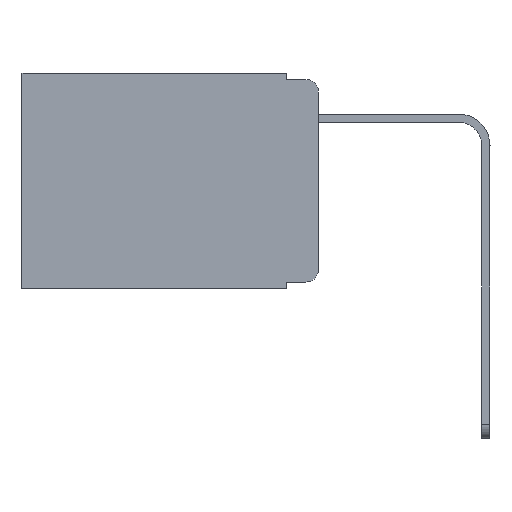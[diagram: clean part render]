
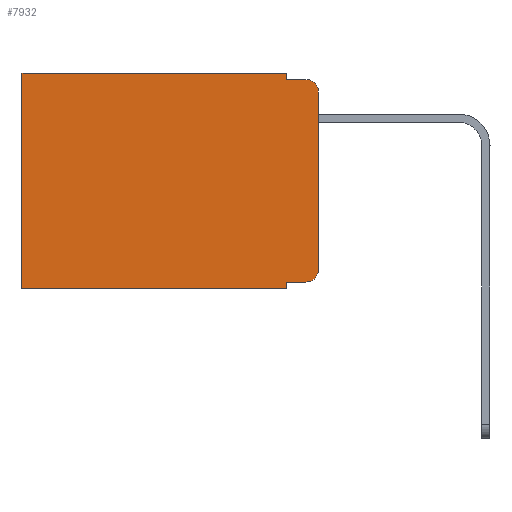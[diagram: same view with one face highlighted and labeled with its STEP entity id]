
A CAD part, left-side view. The second image highlights one B-rep face of the part: STEP entity #7932.
In plain terms, the highlighted planar face has unit normal (-1, 0, 0).
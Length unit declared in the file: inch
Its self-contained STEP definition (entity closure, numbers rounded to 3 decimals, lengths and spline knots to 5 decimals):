
#112 = EDGE_LOOP ( 'NONE', ( #2120, #5656, #2604, #1075, #7360, #4622, #6411, #9965, #1761, #8340 ) ) ;
#137 = DIRECTION ( 'NONE',  ( -1., 0., 0. ) ) ;
#188 = CARTESIAN_POINT ( 'NONE',  ( 0.298, 0.051, -0.333 ) ) ;
#479 = VERTEX_POINT ( 'NONE', #3732 ) ;
#549 = CARTESIAN_POINT ( 'NONE',  ( 0.298, 0.051, -0.01 ) ) ;
#800 = VERTEX_POINT ( 'NONE', #10415 ) ;
#1061 = LINE ( 'NONE', #8242, #6651 ) ;
#1075 = ORIENTED_EDGE ( 'NONE', *, *, #8992, .F. ) ;
#1256 = EDGE_CURVE ( 'NONE', #8599, #2444, #7581, .T. ) ;
#1360 = VERTEX_POINT ( 'NONE', #4017 ) ;
#1378 = AXIS2_PLACEMENT_3D ( 'NONE', #6893, #1524, #9546 ) ;
#1464 = LINE ( 'NONE', #3446, #11587 ) ;
#1524 = DIRECTION ( 'NONE',  ( -1., 0., 0. ) ) ;
#1761 = ORIENTED_EDGE ( 'NONE', *, *, #6581, .T. ) ;
#2064 = EDGE_CURVE ( 'NONE', #1360, #479, #7715, .T. ) ;
#2120 = ORIENTED_EDGE ( 'NONE', *, *, #2064, .F. ) ;
#2444 = VERTEX_POINT ( 'NONE', #5760 ) ;
#2604 = ORIENTED_EDGE ( 'NONE', *, *, #1256, .F. ) ;
#2747 = DIRECTION ( 'NONE',  ( 0., 0., -1. ) ) ;
#2809 = CIRCLE ( 'NONE', #1378, 0.02 ) ;
#3078 = EDGE_CURVE ( 'NONE', #3858, #7158, #6857, .T. ) ;
#3193 = DIRECTION ( 'NONE',  ( 0., -1., 0. ) ) ;
#3205 = CARTESIAN_POINT ( 'NONE',  ( 0.298, 0.051, -0.333 ) ) ;
#3329 = CARTESIAN_POINT ( 'NONE',  ( 0.298, 0.051, 0. ) ) ;
#3446 = CARTESIAN_POINT ( 'NONE',  ( 0.298, 0., 0. ) ) ;
#3451 = DIRECTION ( 'NONE',  ( 0., 0., -1. ) ) ;
#3732 = CARTESIAN_POINT ( 'NONE',  ( 0.298, 0., -0.313 ) ) ;
#3858 = VERTEX_POINT ( 'NONE', #188 ) ;
#4017 = CARTESIAN_POINT ( 'NONE',  ( 0.298, 0., -0.03 ) ) ;
#4024 = CARTESIAN_POINT ( 'NONE',  ( 0.298, 0.051, 0. ) ) ;
#4220 = DIRECTION ( 'NONE',  ( 0., 0., -1. ) ) ;
#4585 = FACE_OUTER_BOUND ( 'NONE', #112, .T. ) ;
#4592 = AXIS2_PLACEMENT_3D ( 'NONE', #9533, #10416, #7659 ) ;
#4622 = ORIENTED_EDGE ( 'NONE', *, *, #8997, .T. ) ;
#4826 = LINE ( 'NONE', #5068, #6928 ) ;
#4845 = VERTEX_POINT ( 'NONE', #10494 ) ;
#5006 = EDGE_CURVE ( 'NONE', #10730, #5674, #1464, .T. ) ;
#5068 = CARTESIAN_POINT ( 'NONE',  ( 0.298, 0., -0.343 ) ) ;
#5199 = VECTOR ( 'NONE', #5952, 39.37008 ) ;
#5656 = ORIENTED_EDGE ( 'NONE', *, *, #10857, .T. ) ;
#5674 = VERTEX_POINT ( 'NONE', #8025 ) ;
#5760 = CARTESIAN_POINT ( 'NONE',  ( 0.298, 0.02, -0.01 ) ) ;
#5952 = DIRECTION ( 'NONE',  ( 0., -1., 0. ) ) ;
#5973 = PLANE ( 'NONE',  #4592 ) ;
#6411 = ORIENTED_EDGE ( 'NONE', *, *, #9821, .F. ) ;
#6581 = EDGE_CURVE ( 'NONE', #3858, #4845, #7562, .T. ) ;
#6651 = VECTOR ( 'NONE', #2747, 39.37008 ) ;
#6857 = LINE ( 'NONE', #4024, #9399 ) ;
#6893 = CARTESIAN_POINT ( 'NONE',  ( 0.298, 0.02, -0.313 ) ) ;
#6928 = VECTOR ( 'NONE', #11342, 39.37008 ) ;
#6968 = CARTESIAN_POINT ( 'NONE',  ( 0.298, 0.051, -0.343 ) ) ;
#7158 = VERTEX_POINT ( 'NONE', #6968 ) ;
#7360 = ORIENTED_EDGE ( 'NONE', *, *, #5006, .T. ) ;
#7562 = LINE ( 'NONE', #3205, #5199 ) ;
#7581 = LINE ( 'NONE', #549, #8562 ) ;
#7645 = VECTOR ( 'NONE', #4220, 39.37008 ) ;
#7659 = DIRECTION ( 'NONE',  ( 0., 0., -1. ) ) ;
#7715 = LINE ( 'NONE', #11589, #8263 ) ;
#7932 = ADVANCED_FACE ( 'NONE', ( #4585 ), #5973, .F. ) ;
#8025 = CARTESIAN_POINT ( 'NONE',  ( 0.298, 0.473, 0. ) ) ;
#8183 = CARTESIAN_POINT ( 'NONE',  ( 0.298, 0.02, -0.03 ) ) ;
#8242 = CARTESIAN_POINT ( 'NONE',  ( 0.298, 0.473, 0. ) ) ;
#8263 = VECTOR ( 'NONE', #3451, 39.37008 ) ;
#8340 = ORIENTED_EDGE ( 'NONE', *, *, #11077, .T. ) ;
#8484 = CARTESIAN_POINT ( 'NONE',  ( 0.298, 0.051, -0.01 ) ) ;
#8562 = VECTOR ( 'NONE', #3193, 39.37008 ) ;
#8599 = VERTEX_POINT ( 'NONE', #8484 ) ;
#8734 = DIRECTION ( 'NONE',  ( 0., 0., -1. ) ) ;
#8992 = EDGE_CURVE ( 'NONE', #10730, #8599, #9781, .T. ) ;
#8997 = EDGE_CURVE ( 'NONE', #5674, #800, #1061, .T. ) ;
#9399 = VECTOR ( 'NONE', #8734, 39.37008 ) ;
#9533 = CARTESIAN_POINT ( 'NONE',  ( 0.298, 0., 0. ) ) ;
#9546 = DIRECTION ( 'NONE',  ( 0., 0., -1. ) ) ;
#9781 = LINE ( 'NONE', #11107, #7645 ) ;
#9821 = EDGE_CURVE ( 'NONE', #7158, #800, #4826, .T. ) ;
#9965 = ORIENTED_EDGE ( 'NONE', *, *, #3078, .F. ) ;
#10415 = CARTESIAN_POINT ( 'NONE',  ( 0.298, 0.473, -0.343 ) ) ;
#10416 = DIRECTION ( 'NONE',  ( 1., 0., 0. ) ) ;
#10494 = CARTESIAN_POINT ( 'NONE',  ( 0.298, 0.02, -0.333 ) ) ;
#10679 = DIRECTION ( 'NONE',  ( 0., 1., 0. ) ) ;
#10730 = VERTEX_POINT ( 'NONE', #3329 ) ;
#10857 = EDGE_CURVE ( 'NONE', #1360, #2444, #10966, .T. ) ;
#10966 = CIRCLE ( 'NONE', #11389, 0.02 ) ;
#10970 = DIRECTION ( 'NONE',  ( 0., 0., -1. ) ) ;
#11077 = EDGE_CURVE ( 'NONE', #4845, #479, #2809, .T. ) ;
#11107 = CARTESIAN_POINT ( 'NONE',  ( 0.298, 0.051, 0. ) ) ;
#11342 = DIRECTION ( 'NONE',  ( 0., 1., 0. ) ) ;
#11389 = AXIS2_PLACEMENT_3D ( 'NONE', #8183, #137, #10970 ) ;
#11587 = VECTOR ( 'NONE', #10679, 39.37008 ) ;
#11589 = CARTESIAN_POINT ( 'NONE',  ( 0.298, 0., 0. ) ) ;
